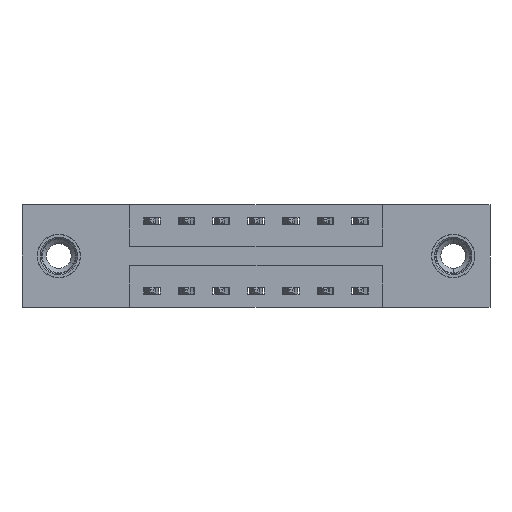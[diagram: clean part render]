
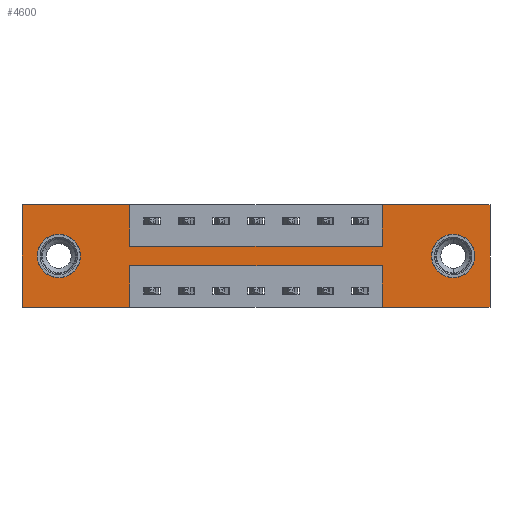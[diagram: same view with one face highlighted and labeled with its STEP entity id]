
A CAD part, front view. The second image highlights one B-rep face of the part: STEP entity #4600.
In plain terms, the highlighted planar face has unit normal (0, -1, 0).
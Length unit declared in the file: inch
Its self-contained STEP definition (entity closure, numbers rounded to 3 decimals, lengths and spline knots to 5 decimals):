
#105 = VECTOR ( 'NONE', #733, 39.37008 ) ;
#129 = CARTESIAN_POINT ( 'NONE',  ( 0.1325, 0., -0.107 ) ) ;
#131 = DIRECTION ( 'NONE',  ( 0., 0., 1. ) ) ;
#135 = CARTESIAN_POINT ( 'NONE',  ( 0.3875, 0., -0.37 ) ) ;
#533 = DIRECTION ( 'NONE',  ( 0., 0., 1. ) ) ;
#632 = ORIENTED_EDGE ( 'NONE', *, *, #1432, .T. ) ;
#675 = CARTESIAN_POINT ( 'NONE',  ( 1.685, 0., 0. ) ) ;
#733 = DIRECTION ( 'NONE',  ( -1., 0., 0. ) ) ;
#740 = EDGE_CURVE ( 'NONE', #7095, #4451, #3381, .T. ) ;
#757 = DIRECTION ( 'NONE',  ( -1., 0., 0. ) ) ;
#764 = ORIENTED_EDGE ( 'NONE', *, *, #5165, .F. ) ;
#929 = CARTESIAN_POINT ( 'NONE',  ( 1.5525, 0., -0.107 ) ) ;
#1210 = FACE_BOUND ( 'NONE', #5979, .T. ) ;
#1228 = VERTEX_POINT ( 'NONE', #7363 ) ;
#1239 = CIRCLE ( 'NONE', #3122, 0.078 ) ;
#1307 = CIRCLE ( 'NONE', #6726, 0.078 ) ;
#1424 = AXIS2_PLACEMENT_3D ( 'NONE', #5176, #5228, #10000 ) ;
#1432 = EDGE_CURVE ( 'NONE', #8603, #9119, #1239, .T. ) ;
#1691 = VERTEX_POINT ( 'NONE', #129 ) ;
#1715 = VERTEX_POINT ( 'NONE', #3456 ) ;
#1778 = DIRECTION ( 'NONE',  ( -1., 0., 0. ) ) ;
#1791 = CARTESIAN_POINT ( 'NONE',  ( 1.2975, 0., -0.37 ) ) ;
#1827 = DIRECTION ( 'NONE',  ( 0., 0., -1. ) ) ;
#1865 = VECTOR ( 'NONE', #1827, 39.37008 ) ;
#1907 = FACE_BOUND ( 'NONE', #7124, .T. ) ;
#1928 = EDGE_CURVE ( 'NONE', #1715, #2084, #6177, .T. ) ;
#1973 = DIRECTION ( 'NONE',  ( 0., 0., -1. ) ) ;
#2026 = CARTESIAN_POINT ( 'NONE',  ( 0.1325, 0., -0.185 ) ) ;
#2064 = CIRCLE ( 'NONE', #5135, 0.078 ) ;
#2071 = CARTESIAN_POINT ( 'NONE',  ( 0., 0., 0. ) ) ;
#2084 = VERTEX_POINT ( 'NONE', #2628 ) ;
#2135 = ORIENTED_EDGE ( 'NONE', *, *, #5085, .F. ) ;
#2226 = ORIENTED_EDGE ( 'NONE', *, *, #7573, .F. ) ;
#2242 = CARTESIAN_POINT ( 'NONE',  ( 0.1325, 0., -0.263 ) ) ;
#2492 = CIRCLE ( 'NONE', #8442, 0.078 ) ;
#2628 = CARTESIAN_POINT ( 'NONE',  ( 1.2975, 0., 0. ) ) ;
#2754 = ORIENTED_EDGE ( 'NONE', *, *, #6393, .F. ) ;
#2816 = LINE ( 'NONE', #6909, #8467 ) ;
#2820 = EDGE_CURVE ( 'NONE', #9119, #8603, #2064, .T. ) ;
#2875 = PLANE ( 'NONE',  #1424 ) ;
#2943 = VECTOR ( 'NONE', #757, 39.37008 ) ;
#3009 = CARTESIAN_POINT ( 'NONE',  ( 0., 0., -0.37 ) ) ;
#3013 = ORIENTED_EDGE ( 'NONE', *, *, #740, .F. ) ;
#3122 = AXIS2_PLACEMENT_3D ( 'NONE', #9360, #6031, #10109 ) ;
#3192 = EDGE_CURVE ( 'NONE', #4664, #3286, #7506, .T. ) ;
#3286 = VERTEX_POINT ( 'NONE', #9204 ) ;
#3379 = VECTOR ( 'NONE', #5919, 39.37008 ) ;
#3381 = LINE ( 'NONE', #8273, #1865 ) ;
#3439 = VERTEX_POINT ( 'NONE', #7935 ) ;
#3448 = CARTESIAN_POINT ( 'NONE',  ( 0.3875, 0., -0.22 ) ) ;
#3456 = CARTESIAN_POINT ( 'NONE',  ( 1.2975, 0., -0.15 ) ) ;
#3517 = FACE_OUTER_BOUND ( 'NONE', #3910, .T. ) ;
#3731 = EDGE_CURVE ( 'NONE', #6314, #1228, #4358, .T. ) ;
#3910 = EDGE_LOOP ( 'NONE', ( #3013, #4924, #6213, #764, #2226, #2135, #9296, #2754, #7806, #10057, #9446, #7258 ) ) ;
#3994 = ORIENTED_EDGE ( 'NONE', *, *, #2820, .T. ) ;
#4093 = EDGE_CURVE ( 'NONE', #1228, #7095, #4839, .T. ) ;
#4249 = ORIENTED_EDGE ( 'NONE', *, *, #6307, .T. ) ;
#4358 = LINE ( 'NONE', #1791, #9896 ) ;
#4372 = VECTOR ( 'NONE', #6711, 39.37008 ) ;
#4451 = VERTEX_POINT ( 'NONE', #135 ) ;
#4600 = ADVANCED_FACE ( 'NONE', ( #1210, #1907, #3517 ), #2875, .T. ) ;
#4664 = VERTEX_POINT ( 'NONE', #2071 ) ;
#4704 = DIRECTION ( 'NONE',  ( 1., 0., 0. ) ) ;
#4754 = LINE ( 'NONE', #6402, #8539 ) ;
#4839 = LINE ( 'NONE', #5795, #105 ) ;
#4924 = ORIENTED_EDGE ( 'NONE', *, *, #4093, .F. ) ;
#5059 = DIRECTION ( 'NONE',  ( 0., 0., 1. ) ) ;
#5085 = EDGE_CURVE ( 'NONE', #2084, #9500, #4754, .T. ) ;
#5135 = AXIS2_PLACEMENT_3D ( 'NONE', #10054, #9258, #1973 ) ;
#5165 = EDGE_CURVE ( 'NONE', #10388, #6314, #8631, .T. ) ;
#5176 = CARTESIAN_POINT ( 'NONE',  ( 0., 0., -0.37 ) ) ;
#5225 = DIRECTION ( 'NONE',  ( 1., 0., 0. ) ) ;
#5228 = DIRECTION ( 'NONE',  ( 0., -1., 0. ) ) ;
#5264 = CARTESIAN_POINT ( 'NONE',  ( 1.685, 0., -0.37 ) ) ;
#5663 = VECTOR ( 'NONE', #5225, 39.37008 ) ;
#5795 = CARTESIAN_POINT ( 'NONE',  ( 0.3875, 0., -0.22 ) ) ;
#5811 = LINE ( 'NONE', #8347, #6079 ) ;
#5919 = DIRECTION ( 'NONE',  ( 0., 0., -1. ) ) ;
#5979 = EDGE_LOOP ( 'NONE', ( #632, #3994 ) ) ;
#6031 = DIRECTION ( 'NONE',  ( 0., 1., 0. ) ) ;
#6070 = DIRECTION ( 'NONE',  ( 0., 0., -1. ) ) ;
#6079 = VECTOR ( 'NONE', #6752, 39.37008 ) ;
#6084 = DIRECTION ( 'NONE',  ( 0., 0., 1. ) ) ;
#6177 = LINE ( 'NONE', #8974, #9559 ) ;
#6213 = ORIENTED_EDGE ( 'NONE', *, *, #3731, .F. ) ;
#6307 = EDGE_CURVE ( 'NONE', #9198, #1691, #2492, .T. ) ;
#6314 = VERTEX_POINT ( 'NONE', #9049 ) ;
#6393 = EDGE_CURVE ( 'NONE', #3439, #1715, #5811, .T. ) ;
#6402 = CARTESIAN_POINT ( 'NONE',  ( 0., 0., 0. ) ) ;
#6594 = DIRECTION ( 'NONE',  ( 0., 1., 0. ) ) ;
#6711 = DIRECTION ( 'NONE',  ( 0., 0., 1. ) ) ;
#6726 = AXIS2_PLACEMENT_3D ( 'NONE', #2026, #10380, #6084 ) ;
#6752 = DIRECTION ( 'NONE',  ( 1., 0., 0. ) ) ;
#6909 = CARTESIAN_POINT ( 'NONE',  ( 0.3875, 0., 0. ) ) ;
#7095 = VERTEX_POINT ( 'NONE', #3448 ) ;
#7124 = EDGE_LOOP ( 'NONE', ( #9147, #4249 ) ) ;
#7258 = ORIENTED_EDGE ( 'NONE', *, *, #8473, .F. ) ;
#7363 = CARTESIAN_POINT ( 'NONE',  ( 1.2975, 0., -0.22 ) ) ;
#7506 = LINE ( 'NONE', #8449, #5663 ) ;
#7573 = EDGE_CURVE ( 'NONE', #9500, #10388, #8346, .T. ) ;
#7733 = EDGE_CURVE ( 'NONE', #3286, #3439, #2816, .T. ) ;
#7806 = ORIENTED_EDGE ( 'NONE', *, *, #7733, .F. ) ;
#7921 = LINE ( 'NONE', #9557, #9629 ) ;
#7935 = CARTESIAN_POINT ( 'NONE',  ( 0.3875, 0., -0.15 ) ) ;
#8273 = CARTESIAN_POINT ( 'NONE',  ( 0.3875, 0., -0.37 ) ) ;
#8346 = LINE ( 'NONE', #9784, #3379 ) ;
#8347 = CARTESIAN_POINT ( 'NONE',  ( 0.3875, 0., -0.15 ) ) ;
#8442 = AXIS2_PLACEMENT_3D ( 'NONE', #9107, #6594, #131 ) ;
#8449 = CARTESIAN_POINT ( 'NONE',  ( 0., 0., 0. ) ) ;
#8459 = CARTESIAN_POINT ( 'NONE',  ( 1.5525, 0., -0.263 ) ) ;
#8467 = VECTOR ( 'NONE', #6070, 39.37008 ) ;
#8473 = EDGE_CURVE ( 'NONE', #4451, #9380, #7921, .T. ) ;
#8539 = VECTOR ( 'NONE', #4704, 39.37008 ) ;
#8603 = VERTEX_POINT ( 'NONE', #929 ) ;
#8631 = LINE ( 'NONE', #8841, #2943 ) ;
#8841 = CARTESIAN_POINT ( 'NONE',  ( 0., 0., -0.37 ) ) ;
#8974 = CARTESIAN_POINT ( 'NONE',  ( 1.2975, 0., 0. ) ) ;
#9049 = CARTESIAN_POINT ( 'NONE',  ( 1.2975, 0., -0.37 ) ) ;
#9107 = CARTESIAN_POINT ( 'NONE',  ( 0.1325, 0., -0.185 ) ) ;
#9116 = CARTESIAN_POINT ( 'NONE',  ( 0., 0., 0. ) ) ;
#9119 = VERTEX_POINT ( 'NONE', #8459 ) ;
#9139 = EDGE_CURVE ( 'NONE', #9380, #4664, #9904, .T. ) ;
#9147 = ORIENTED_EDGE ( 'NONE', *, *, #9266, .T. ) ;
#9198 = VERTEX_POINT ( 'NONE', #2242 ) ;
#9204 = CARTESIAN_POINT ( 'NONE',  ( 0.3875, 0., 0. ) ) ;
#9258 = DIRECTION ( 'NONE',  ( 0., 1., 0. ) ) ;
#9266 = EDGE_CURVE ( 'NONE', #1691, #9198, #1307, .T. ) ;
#9296 = ORIENTED_EDGE ( 'NONE', *, *, #1928, .F. ) ;
#9360 = CARTESIAN_POINT ( 'NONE',  ( 1.5525, 0., -0.185 ) ) ;
#9380 = VERTEX_POINT ( 'NONE', #3009 ) ;
#9446 = ORIENTED_EDGE ( 'NONE', *, *, #9139, .F. ) ;
#9500 = VERTEX_POINT ( 'NONE', #675 ) ;
#9557 = CARTESIAN_POINT ( 'NONE',  ( 0., 0., -0.37 ) ) ;
#9559 = VECTOR ( 'NONE', #533, 39.37008 ) ;
#9629 = VECTOR ( 'NONE', #1778, 39.37008 ) ;
#9784 = CARTESIAN_POINT ( 'NONE',  ( 1.685, 0., 0. ) ) ;
#9896 = VECTOR ( 'NONE', #5059, 39.37008 ) ;
#9904 = LINE ( 'NONE', #9116, #4372 ) ;
#10000 = DIRECTION ( 'NONE',  ( 0., 0., -1. ) ) ;
#10054 = CARTESIAN_POINT ( 'NONE',  ( 1.5525, 0., -0.185 ) ) ;
#10057 = ORIENTED_EDGE ( 'NONE', *, *, #3192, .F. ) ;
#10109 = DIRECTION ( 'NONE',  ( 0., 0., -1. ) ) ;
#10380 = DIRECTION ( 'NONE',  ( 0., 1., 0. ) ) ;
#10388 = VERTEX_POINT ( 'NONE', #5264 ) ;
